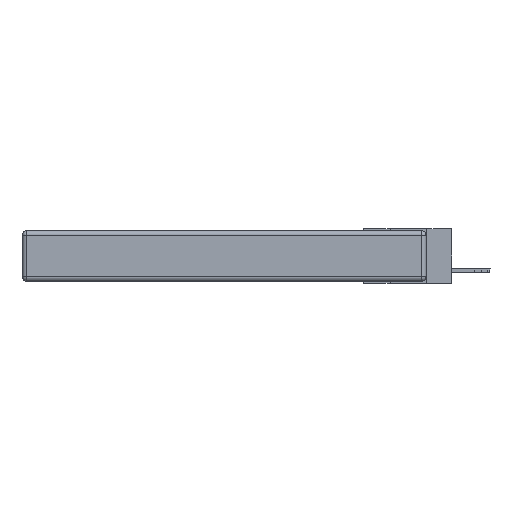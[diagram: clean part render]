
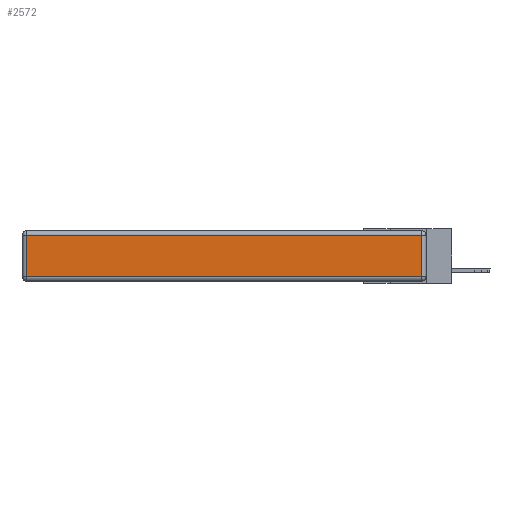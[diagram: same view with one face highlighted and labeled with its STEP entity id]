
A CAD part, left-side view. The second image highlights one B-rep face of the part: STEP entity #2572.
In plain terms, the highlighted planar face has unit normal (-1, 0, 0).
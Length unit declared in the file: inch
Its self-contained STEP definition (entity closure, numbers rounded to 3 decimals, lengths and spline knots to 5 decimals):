
#1434 = DIRECTION ( 'NONE',  ( 0., 1., 0. ) ) ;
#1704 = EDGE_CURVE ( 'NONE', #8324, #26573, #14132, .T. ) ;
#2572 = ADVANCED_FACE ( 'NONE', ( #24079 ), #7893, .T. ) ;
#3506 = DIRECTION ( 'NONE',  ( 0., 0., 1. ) ) ;
#3545 = EDGE_CURVE ( 'NONE', #7788, #27015, #5674, .T. ) ;
#4138 = DIRECTION ( 'NONE',  ( 0., -1., 0. ) ) ;
#4297 = ORIENTED_EDGE ( 'NONE', *, *, #16570, .T. ) ;
#5674 = LINE ( 'NONE', #12386, #10980 ) ;
#6739 = ORIENTED_EDGE ( 'NONE', *, *, #10339, .T. ) ;
#6851 = ORIENTED_EDGE ( 'NONE', *, *, #3545, .T. ) ;
#7788 = VERTEX_POINT ( 'NONE', #25496 ) ;
#7893 = PLANE ( 'NONE',  #18141 ) ;
#8311 = CARTESIAN_POINT ( 'NONE',  ( 0., 0.03, -0.313 ) ) ;
#8324 = VERTEX_POINT ( 'NONE', #9529 ) ;
#8445 = DIRECTION ( 'NONE',  ( 0., 0., -1. ) ) ;
#9529 = CARTESIAN_POINT ( 'NONE',  ( 0., 2.72, -0.313 ) ) ;
#10339 = EDGE_CURVE ( 'NONE', #27015, #8324, #24828, .T. ) ;
#10980 = VECTOR ( 'NONE', #1434, 39.37008 ) ;
#12123 = VECTOR ( 'NONE', #4138, 39.37008 ) ;
#12386 = CARTESIAN_POINT ( 'NONE',  ( 0., 2.75, -0.03 ) ) ;
#12525 = DIRECTION ( 'NONE',  ( -1., 0., 0. ) ) ;
#12966 = VECTOR ( 'NONE', #8445, 39.37008 ) ;
#14132 = LINE ( 'NONE', #14591, #12123 ) ;
#14591 = CARTESIAN_POINT ( 'NONE',  ( 0., 0., -0.313 ) ) ;
#16570 = EDGE_CURVE ( 'NONE', #26573, #7788, #25432, .T. ) ;
#18141 = AXIS2_PLACEMENT_3D ( 'NONE', #22547, #12525, #19572 ) ;
#19154 = VECTOR ( 'NONE', #3506, 39.37008 ) ;
#19572 = DIRECTION ( 'NONE',  ( 0., 0., 1. ) ) ;
#20732 = ORIENTED_EDGE ( 'NONE', *, *, #1704, .T. ) ;
#21075 = CARTESIAN_POINT ( 'NONE',  ( 0., 2.72, -0.343 ) ) ;
#22447 = CARTESIAN_POINT ( 'NONE',  ( 0., 0.03, -0.343 ) ) ;
#22547 = CARTESIAN_POINT ( 'NONE',  ( 0., 0., -0.343 ) ) ;
#23078 = EDGE_LOOP ( 'NONE', ( #20732, #4297, #6851, #6739 ) ) ;
#23280 = CARTESIAN_POINT ( 'NONE',  ( 0., 2.72, -0.03 ) ) ;
#24079 = FACE_OUTER_BOUND ( 'NONE', #23078, .T. ) ;
#24828 = LINE ( 'NONE', #21075, #12966 ) ;
#25432 = LINE ( 'NONE', #22447, #19154 ) ;
#25496 = CARTESIAN_POINT ( 'NONE',  ( 0., 0.03, -0.03 ) ) ;
#26573 = VERTEX_POINT ( 'NONE', #8311 ) ;
#27015 = VERTEX_POINT ( 'NONE', #23280 ) ;
